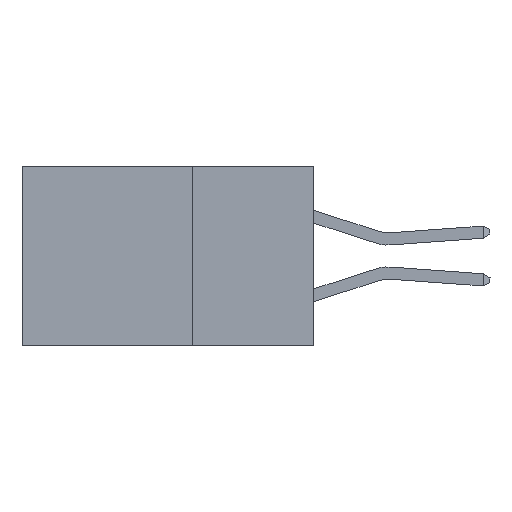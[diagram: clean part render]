
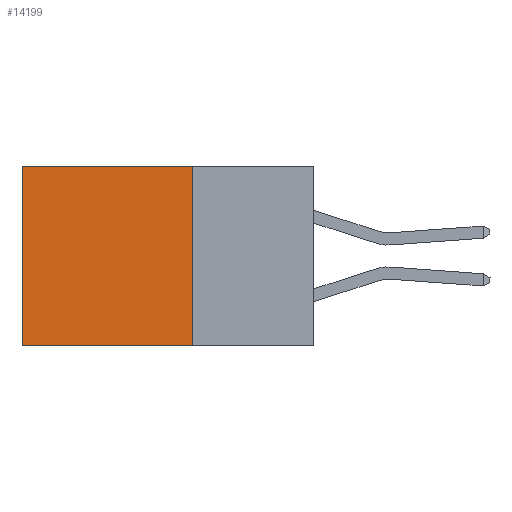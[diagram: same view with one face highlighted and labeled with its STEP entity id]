
A CAD part, left-side view. The second image highlights one B-rep face of the part: STEP entity #14199.
In plain terms, the highlighted planar face has unit normal (-1, 0, 0).
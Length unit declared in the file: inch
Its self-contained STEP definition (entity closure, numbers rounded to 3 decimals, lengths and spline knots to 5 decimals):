
#3 = DIRECTION ( 'NONE',  ( 0., 0., -1. ) ) ;
#374 = LINE ( 'NONE', #11147, #4727 ) ;
#978 = CARTESIAN_POINT ( 'NONE',  ( 0.2875, 0.6, -0.37 ) ) ;
#1919 = VERTEX_POINT ( 'NONE', #4428 ) ;
#2307 = CARTESIAN_POINT ( 'NONE',  ( 0.2875, 0.25, 0. ) ) ;
#2412 = ORIENTED_EDGE ( 'NONE', *, *, #11996, .T. ) ;
#3327 = DIRECTION ( 'NONE',  ( 0., 1., 0. ) ) ;
#3623 = PLANE ( 'NONE',  #14550 ) ;
#3683 = DIRECTION ( 'NONE',  ( 1., 0., 0. ) ) ;
#3854 = CARTESIAN_POINT ( 'NONE',  ( 0.2875, 0.6, 0. ) ) ;
#4330 = CARTESIAN_POINT ( 'NONE',  ( 0.2875, 0.25, -0.37 ) ) ;
#4428 = CARTESIAN_POINT ( 'NONE',  ( 0.2875, 0.25, 0. ) ) ;
#4727 = VECTOR ( 'NONE', #14651, 39.37008 ) ;
#4741 = LINE ( 'NONE', #6548, #14723 ) ;
#6493 = LINE ( 'NONE', #13034, #16686 ) ;
#6548 = CARTESIAN_POINT ( 'NONE',  ( 0.2875, 0.25, 0. ) ) ;
#7322 = EDGE_CURVE ( 'NONE', #1919, #9601, #16892, .T. ) ;
#8234 = EDGE_CURVE ( 'NONE', #16669, #14137, #374, .T. ) ;
#8400 = CARTESIAN_POINT ( 'NONE',  ( 0.2875, 0.25, 0. ) ) ;
#9601 = VERTEX_POINT ( 'NONE', #4330 ) ;
#9669 = ORIENTED_EDGE ( 'NONE', *, *, #8234, .T. ) ;
#10726 = EDGE_LOOP ( 'NONE', ( #9669, #12370, #12295, #2412 ) ) ;
#11147 = CARTESIAN_POINT ( 'NONE',  ( 0.2875, 0.6, 0. ) ) ;
#11739 = EDGE_CURVE ( 'NONE', #9601, #14137, #6493, .T. ) ;
#11996 = EDGE_CURVE ( 'NONE', #1919, #16669, #4741, .T. ) ;
#12009 = DIRECTION ( 'NONE',  ( 0., 1., 0. ) ) ;
#12295 = ORIENTED_EDGE ( 'NONE', *, *, #7322, .F. ) ;
#12370 = ORIENTED_EDGE ( 'NONE', *, *, #11739, .F. ) ;
#13034 = CARTESIAN_POINT ( 'NONE',  ( 0.2875, 0.25, -0.37 ) ) ;
#13391 = DIRECTION ( 'NONE',  ( 0., 0., -1. ) ) ;
#14137 = VERTEX_POINT ( 'NONE', #978 ) ;
#14199 = ADVANCED_FACE ( 'NONE', ( #16147 ), #3623, .F. ) ;
#14550 = AXIS2_PLACEMENT_3D ( 'NONE', #2307, #3683, #13391 ) ;
#14651 = DIRECTION ( 'NONE',  ( 0., 0., -1. ) ) ;
#14723 = VECTOR ( 'NONE', #12009, 39.37008 ) ;
#16147 = FACE_OUTER_BOUND ( 'NONE', #10726, .T. ) ;
#16669 = VERTEX_POINT ( 'NONE', #3854 ) ;
#16686 = VECTOR ( 'NONE', #3327, 39.37008 ) ;
#16892 = LINE ( 'NONE', #8400, #17093 ) ;
#17093 = VECTOR ( 'NONE', #3, 39.37008 ) ;
